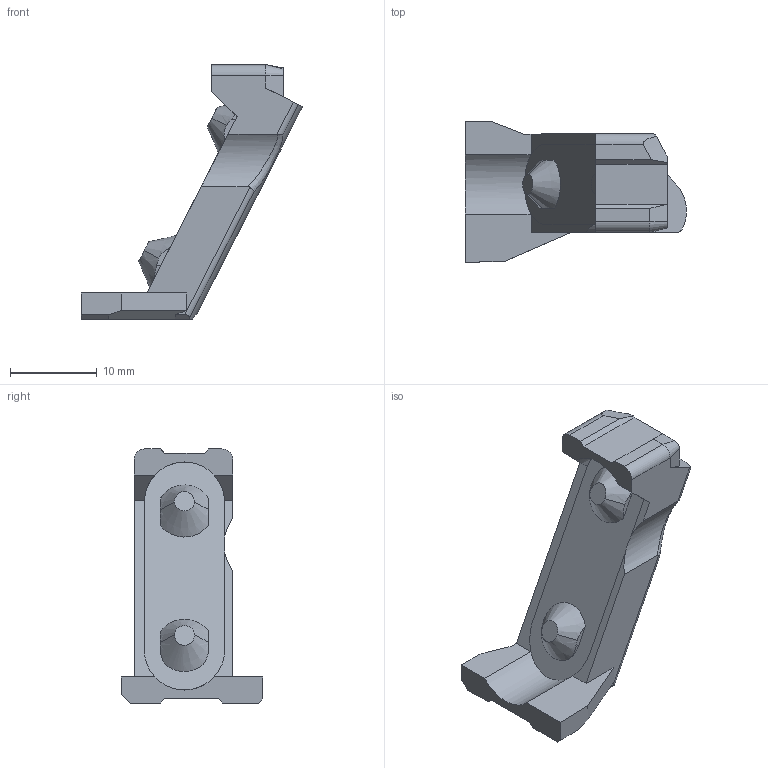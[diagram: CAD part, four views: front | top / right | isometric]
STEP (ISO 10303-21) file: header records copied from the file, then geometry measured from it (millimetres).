
FILE_DESCRIPTION(/* description */ (''),/* implementation_level */ '2;1');
FILE_NAME(/* name */ 'M&P Follower.step',/* time_stamp */ '2023-01-05T17:02:21-06:00',/* author */ (''),/* organization */ (''),/* preprocessor_version */ 'ST-DEVELOPER v19.2',/* originating_system */ 'Autodesk Translation Framework v11.17.0.187',/* authorisation */ '');
FILE_SCHEMA (('AUTOMOTIVE_DESIGN { 1 0 10303 214 3 1 1 }'));
Length unit declared in the file: millimetre
Products named in the file (1): M&P Follower V1.1
Bounding box: 25.45 x 16.23 x 29.25 mm (x, y, z)
Volume: 1909.3 mm3; surface area: 1523.1 mm2
Topology: 1 solids, 1 shells, 67 faces, 181 edges, 118 vertices
Faces by surface type: plane 45, cylinder 15, bspline 4, cone 3
Entity records: 2537 total; most frequent: CARTESIAN_POINT 856, ORIENTED_EDGE 362, DIRECTION 319, EDGE_CURVE 181, VERTEX_POINT 118, LINE 111, VECTOR 111, AXIS2_PLACEMENT_3D 104
